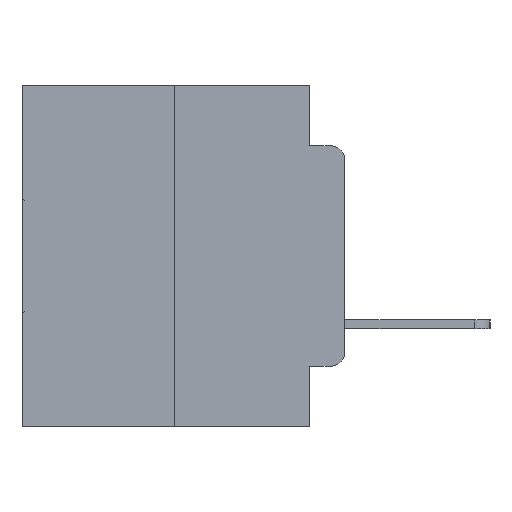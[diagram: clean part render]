
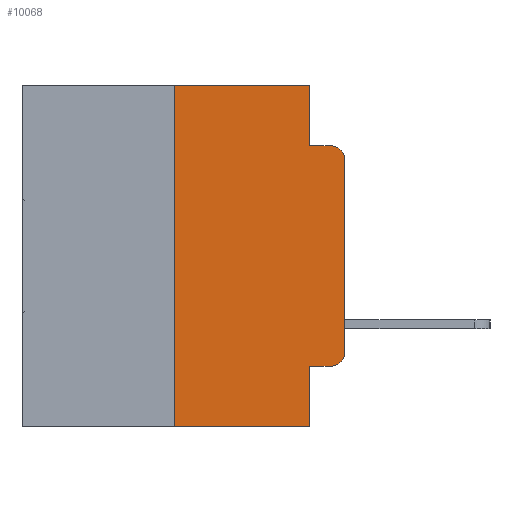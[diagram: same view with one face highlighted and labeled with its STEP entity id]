
A CAD part, left-side view. The second image highlights one B-rep face of the part: STEP entity #10068.
In plain terms, the highlighted planar face has unit normal (-1, 0, 0).
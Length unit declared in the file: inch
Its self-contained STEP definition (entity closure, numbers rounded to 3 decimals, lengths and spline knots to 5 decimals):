
#515 = EDGE_CURVE ( 'NONE', #18830, #4908, #15211, .T. ) ;
#842 = DIRECTION ( 'NONE',  ( 0., 0., -1. ) ) ;
#1422 = DIRECTION ( 'NONE',  ( 0., 0., -1. ) ) ;
#1608 = ORIENTED_EDGE ( 'NONE', *, *, #8350, .F. ) ;
#2530 = EDGE_CURVE ( 'NONE', #3890, #13050, #21944, .T. ) ;
#3890 = VERTEX_POINT ( 'NONE', #11249 ) ;
#4495 = EDGE_CURVE ( 'NONE', #26930, #24517, #4667, .T. ) ;
#4667 = LINE ( 'NONE', #18725, #19920 ) ;
#4908 = VERTEX_POINT ( 'NONE', #15820 ) ;
#4928 = AXIS2_PLACEMENT_3D ( 'NONE', #25232, #8408, #23301 ) ;
#6300 = VECTOR ( 'NONE', #17596, 39.37008 ) ;
#7170 = CARTESIAN_POINT ( 'NONE',  ( 0., 0.051, -0.5 ) ) ;
#7299 = CARTESIAN_POINT ( 'NONE',  ( 0., 0.02, -0.0885 ) ) ;
#7335 = LINE ( 'NONE', #22216, #17510 ) ;
#7486 = CARTESIAN_POINT ( 'NONE',  ( 0., 0.051, -0.4115 ) ) ;
#7842 = VERTEX_POINT ( 'NONE', #21746 ) ;
#8350 = EDGE_CURVE ( 'NONE', #12124, #18830, #16866, .T. ) ;
#8408 = DIRECTION ( 'NONE',  ( 1., 0., 0. ) ) ;
#8699 = ORIENTED_EDGE ( 'NONE', *, *, #24553, .T. ) ;
#8924 = ORIENTED_EDGE ( 'NONE', *, *, #10017, .T. ) ;
#9013 = LINE ( 'NONE', #25001, #25199 ) ;
#9176 = CARTESIAN_POINT ( 'NONE',  ( 0., 0., 0. ) ) ;
#9408 = VECTOR ( 'NONE', #10925, 39.37008 ) ;
#9626 = ORIENTED_EDGE ( 'NONE', *, *, #2530, .T. ) ;
#9727 = CARTESIAN_POINT ( 'NONE',  ( 0., 0.473, 0. ) ) ;
#10017 = EDGE_CURVE ( 'NONE', #22825, #3890, #26398, .T. ) ;
#10068 = ADVANCED_FACE ( 'NONE', ( #13448 ), #21229, .F. ) ;
#10394 = ORIENTED_EDGE ( 'NONE', *, *, #24714, .F. ) ;
#10925 = DIRECTION ( 'NONE',  ( 0., -1., 0. ) ) ;
#11249 = CARTESIAN_POINT ( 'NONE',  ( 0., 0.02, -0.4115 ) ) ;
#11398 = CIRCLE ( 'NONE', #13889, 0.02 ) ;
#11472 = LINE ( 'NONE', #15469, #6300 ) ;
#11796 = VECTOR ( 'NONE', #23640, 39.37008 ) ;
#12124 = VERTEX_POINT ( 'NONE', #26718 ) ;
#13050 = VERTEX_POINT ( 'NONE', #25893 ) ;
#13448 = FACE_OUTER_BOUND ( 'NONE', #19173, .T. ) ;
#13889 = AXIS2_PLACEMENT_3D ( 'NONE', #26462, #14102, #842 ) ;
#14102 = DIRECTION ( 'NONE',  ( -1., 0., 0. ) ) ;
#14637 = CARTESIAN_POINT ( 'NONE',  ( 0., 0.051, -0.4115 ) ) ;
#15211 = LINE ( 'NONE', #9727, #9408 ) ;
#15280 = AXIS2_PLACEMENT_3D ( 'NONE', #18960, #18873, #18871 ) ;
#15469 = CARTESIAN_POINT ( 'NONE',  ( 0., 0.051, 0. ) ) ;
#15820 = CARTESIAN_POINT ( 'NONE',  ( 0., 0.051, 0. ) ) ;
#16866 = LINE ( 'NONE', #27596, #11796 ) ;
#16882 = DIRECTION ( 'NONE',  ( 0., -1., 0. ) ) ;
#16979 = EDGE_CURVE ( 'NONE', #13050, #7842, #23124, .T. ) ;
#17070 = ORIENTED_EDGE ( 'NONE', *, *, #515, .F. ) ;
#17354 = CARTESIAN_POINT ( 'NONE',  ( 0., 0.051, -0.0885 ) ) ;
#17510 = VECTOR ( 'NONE', #26252, 39.37008 ) ;
#17596 = DIRECTION ( 'NONE',  ( 0., 0., -1. ) ) ;
#18725 = CARTESIAN_POINT ( 'NONE',  ( 0., 0.051, -0.0885 ) ) ;
#18830 = VERTEX_POINT ( 'NONE', #22122 ) ;
#18871 = DIRECTION ( 'NONE',  ( 0., 0., -1. ) ) ;
#18873 = DIRECTION ( 'NONE',  ( -1., 0., 0. ) ) ;
#18960 = CARTESIAN_POINT ( 'NONE',  ( 0., 0.02, -0.3915 ) ) ;
#19068 = ORIENTED_EDGE ( 'NONE', *, *, #23388, .T. ) ;
#19173 = EDGE_LOOP ( 'NONE', ( #19869, #8699, #22346, #10394, #17070, #1608, #19068, #19699, #8924, #9626 ) ) ;
#19568 = DIRECTION ( 'NONE',  ( 0., -1., 0. ) ) ;
#19699 = ORIENTED_EDGE ( 'NONE', *, *, #23232, .F. ) ;
#19869 = ORIENTED_EDGE ( 'NONE', *, *, #16979, .T. ) ;
#19920 = VECTOR ( 'NONE', #19568, 39.37008 ) ;
#20409 = VECTOR ( 'NONE', #16882, 39.37008 ) ;
#21229 = PLANE ( 'NONE',  #4928 ) ;
#21746 = CARTESIAN_POINT ( 'NONE',  ( 0., 0., -0.1085 ) ) ;
#21944 = CIRCLE ( 'NONE', #15280, 0.02 ) ;
#22122 = CARTESIAN_POINT ( 'NONE',  ( 0., 0.25, 0. ) ) ;
#22216 = CARTESIAN_POINT ( 'NONE',  ( 0., 0.473, -0.5 ) ) ;
#22346 = ORIENTED_EDGE ( 'NONE', *, *, #4495, .F. ) ;
#22825 = VERTEX_POINT ( 'NONE', #7486 ) ;
#23124 = LINE ( 'NONE', #9176, #24387 ) ;
#23232 = EDGE_CURVE ( 'NONE', #22825, #25064, #11472, .T. ) ;
#23301 = DIRECTION ( 'NONE',  ( 0., 0., -1. ) ) ;
#23388 = EDGE_CURVE ( 'NONE', #12124, #25064, #7335, .T. ) ;
#23640 = DIRECTION ( 'NONE',  ( 0., 0., 1. ) ) ;
#23993 = DIRECTION ( 'NONE',  ( 0., 0., 1. ) ) ;
#24387 = VECTOR ( 'NONE', #23993, 39.37008 ) ;
#24517 = VERTEX_POINT ( 'NONE', #7299 ) ;
#24553 = EDGE_CURVE ( 'NONE', #7842, #24517, #11398, .T. ) ;
#24714 = EDGE_CURVE ( 'NONE', #4908, #26930, #9013, .T. ) ;
#25001 = CARTESIAN_POINT ( 'NONE',  ( 0., 0.051, 0. ) ) ;
#25064 = VERTEX_POINT ( 'NONE', #7170 ) ;
#25199 = VECTOR ( 'NONE', #1422, 39.37008 ) ;
#25232 = CARTESIAN_POINT ( 'NONE',  ( 0., 0.473, 0. ) ) ;
#25893 = CARTESIAN_POINT ( 'NONE',  ( 0., 0., -0.3915 ) ) ;
#26252 = DIRECTION ( 'NONE',  ( 0., -1., 0. ) ) ;
#26398 = LINE ( 'NONE', #14637, #20409 ) ;
#26462 = CARTESIAN_POINT ( 'NONE',  ( 0., 0.02, -0.1085 ) ) ;
#26718 = CARTESIAN_POINT ( 'NONE',  ( 0., 0.25, -0.5 ) ) ;
#26930 = VERTEX_POINT ( 'NONE', #17354 ) ;
#27596 = CARTESIAN_POINT ( 'NONE',  ( 0., 0.25, 0. ) ) ;
